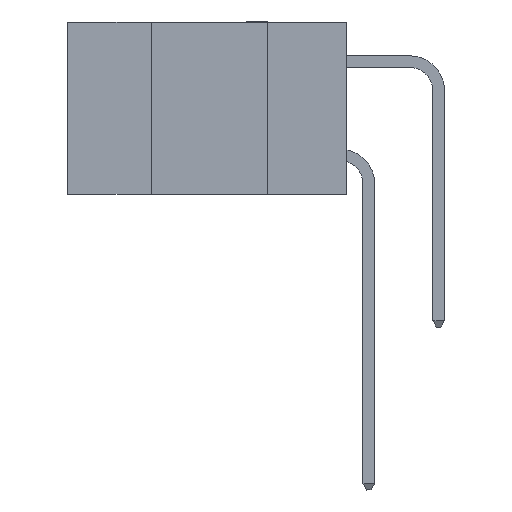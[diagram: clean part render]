
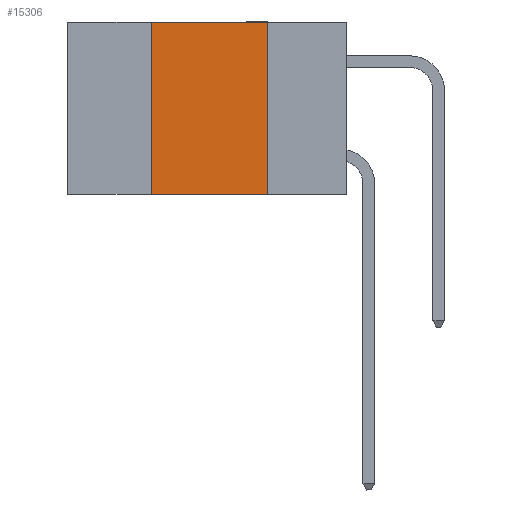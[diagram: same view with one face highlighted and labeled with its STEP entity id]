
A CAD part, left-side view. The second image highlights one B-rep face of the part: STEP entity #15306.
In plain terms, the highlighted planar face has unit normal (-1, 0, 0).
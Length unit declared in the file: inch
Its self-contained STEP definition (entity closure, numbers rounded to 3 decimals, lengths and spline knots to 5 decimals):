
#507 = ORIENTED_EDGE ( 'NONE', *, *, #10024, .F. ) ;
#910 = ORIENTED_EDGE ( 'NONE', *, *, #17561, .F. ) ;
#1135 = VERTEX_POINT ( 'NONE', #12215 ) ;
#1215 = VERTEX_POINT ( 'NONE', #12809 ) ;
#1466 = CARTESIAN_POINT ( 'NONE',  ( 0., 0.6, 0. ) ) ;
#1897 = VERTEX_POINT ( 'NONE', #4687 ) ;
#2328 = CARTESIAN_POINT ( 'NONE',  ( 0., 0.42, -0.37 ) ) ;
#2435 = VECTOR ( 'NONE', #10627, 39.37008 ) ;
#2563 = EDGE_CURVE ( 'NONE', #12286, #1215, #6868, .T. ) ;
#2638 = LINE ( 'NONE', #8863, #5777 ) ;
#3895 = VECTOR ( 'NONE', #11594, 39.37008 ) ;
#4687 = CARTESIAN_POINT ( 'NONE',  ( 0., 0.17, 0. ) ) ;
#5250 = AXIS2_PLACEMENT_3D ( 'NONE', #7008, #14364, #5591 ) ;
#5591 = DIRECTION ( 'NONE',  ( 0., 0., -1. ) ) ;
#5777 = VECTOR ( 'NONE', #17444, 39.37008 ) ;
#6868 = LINE ( 'NONE', #10081, #17970 ) ;
#7008 = CARTESIAN_POINT ( 'NONE',  ( 0., 0.6, 0. ) ) ;
#8383 = LINE ( 'NONE', #10129, #3895 ) ;
#8528 = DIRECTION ( 'NONE',  ( 0., 0., 1. ) ) ;
#8863 = CARTESIAN_POINT ( 'NONE',  ( 0., 0.6, -0.37 ) ) ;
#10024 = EDGE_CURVE ( 'NONE', #1215, #1897, #15629, .T. ) ;
#10081 = CARTESIAN_POINT ( 'NONE',  ( 0., 0.42, 0. ) ) ;
#10129 = CARTESIAN_POINT ( 'NONE',  ( 0., 0.17, 0. ) ) ;
#10627 = DIRECTION ( 'NONE',  ( 0., -1., 0. ) ) ;
#10814 = FACE_OUTER_BOUND ( 'NONE', #12682, .T. ) ;
#11177 = EDGE_CURVE ( 'NONE', #12286, #1135, #2638, .T. ) ;
#11426 = PLANE ( 'NONE',  #5250 ) ;
#11594 = DIRECTION ( 'NONE',  ( 0., 0., -1. ) ) ;
#12215 = CARTESIAN_POINT ( 'NONE',  ( 0., 0.17, -0.37 ) ) ;
#12286 = VERTEX_POINT ( 'NONE', #2328 ) ;
#12682 = EDGE_LOOP ( 'NONE', ( #910, #507, #15553, #16669 ) ) ;
#12809 = CARTESIAN_POINT ( 'NONE',  ( 0., 0.42, 0. ) ) ;
#14364 = DIRECTION ( 'NONE',  ( 1., 0., 0. ) ) ;
#15306 = ADVANCED_FACE ( 'NONE', ( #10814 ), #11426, .F. ) ;
#15553 = ORIENTED_EDGE ( 'NONE', *, *, #2563, .F. ) ;
#15629 = LINE ( 'NONE', #1466, #2435 ) ;
#16669 = ORIENTED_EDGE ( 'NONE', *, *, #11177, .T. ) ;
#17444 = DIRECTION ( 'NONE',  ( 0., -1., 0. ) ) ;
#17561 = EDGE_CURVE ( 'NONE', #1897, #1135, #8383, .T. ) ;
#17970 = VECTOR ( 'NONE', #8528, 39.37008 ) ;
